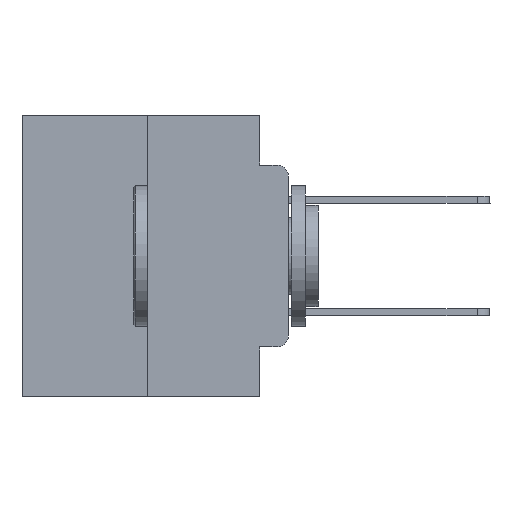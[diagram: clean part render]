
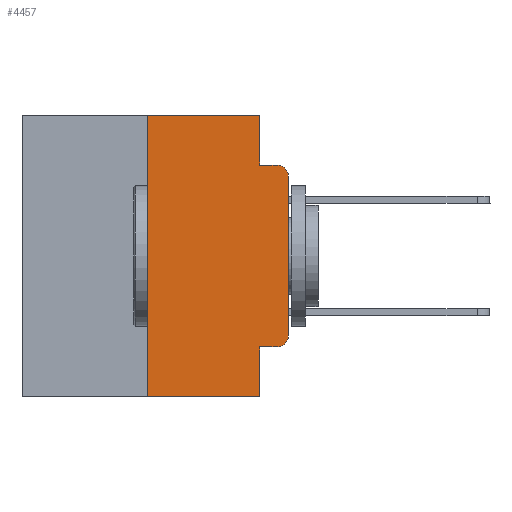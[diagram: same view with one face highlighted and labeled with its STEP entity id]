
A CAD part, left-side view. The second image highlights one B-rep face of the part: STEP entity #4457.
In plain terms, the highlighted planar face has unit normal (-1, 0, 0).
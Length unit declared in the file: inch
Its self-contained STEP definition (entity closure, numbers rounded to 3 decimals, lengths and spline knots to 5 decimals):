
#170 = VECTOR ( 'NONE', #10682, 39.37008 ) ;
#253 = CARTESIAN_POINT ( 'NONE',  ( 0., 0.051, -0.0885 ) ) ;
#426 = CIRCLE ( 'NONE', #10935, 0.02 ) ;
#489 = DIRECTION ( 'NONE',  ( 0., 0., -1. ) ) ;
#490 = ORIENTED_EDGE ( 'NONE', *, *, #3963, .F. ) ;
#1934 = ORIENTED_EDGE ( 'NONE', *, *, #18304, .F. ) ;
#2082 = FACE_OUTER_BOUND ( 'NONE', #13481, .T. ) ;
#2412 = LINE ( 'NONE', #6698, #9205 ) ;
#3065 = DIRECTION ( 'NONE',  ( 0., -1., 0. ) ) ;
#3871 = CARTESIAN_POINT ( 'NONE',  ( 0., 0.051, -0.4115 ) ) ;
#3873 = DIRECTION ( 'NONE',  ( 0., 0., 1. ) ) ;
#3963 = EDGE_CURVE ( 'NONE', #28118, #27911, #18214, .T. ) ;
#4024 = CARTESIAN_POINT ( 'NONE',  ( 0., 0.02, -0.0885 ) ) ;
#4457 = ADVANCED_FACE ( 'NONE', ( #2082 ), #15470, .F. ) ;
#4655 = DIRECTION ( 'NONE',  ( 0., -1., 0. ) ) ;
#4785 = EDGE_CURVE ( 'NONE', #17108, #12115, #7833, .T. ) ;
#4813 = DIRECTION ( 'NONE',  ( 0., 0., -1. ) ) ;
#5510 = ORIENTED_EDGE ( 'NONE', *, *, #4785, .T. ) ;
#5801 = VECTOR ( 'NONE', #9537, 39.37008 ) ;
#5929 = CARTESIAN_POINT ( 'NONE',  ( 0., 0.051, -0.4115 ) ) ;
#5963 = CARTESIAN_POINT ( 'NONE',  ( 0., 0.02, -0.1085 ) ) ;
#6230 = DIRECTION ( 'NONE',  ( 0., 0., -1. ) ) ;
#6346 = LINE ( 'NONE', #23886, #170 ) ;
#6427 = CARTESIAN_POINT ( 'NONE',  ( 0., 0., -0.3915 ) ) ;
#6698 = CARTESIAN_POINT ( 'NONE',  ( 0., 0.051, 0. ) ) ;
#7161 = CARTESIAN_POINT ( 'NONE',  ( 0., 0., 0. ) ) ;
#7327 = EDGE_CURVE ( 'NONE', #15707, #21392, #11937, .T. ) ;
#7483 = VECTOR ( 'NONE', #16942, 39.37008 ) ;
#7833 = LINE ( 'NONE', #7161, #5801 ) ;
#8569 = ORIENTED_EDGE ( 'NONE', *, *, #23806, .F. ) ;
#8581 = VECTOR ( 'NONE', #4655, 39.37008 ) ;
#9099 = CARTESIAN_POINT ( 'NONE',  ( 0., 0.473, 0. ) ) ;
#9205 = VECTOR ( 'NONE', #489, 39.37008 ) ;
#9537 = DIRECTION ( 'NONE',  ( 0., 0., 1. ) ) ;
#9741 = VECTOR ( 'NONE', #12389, 39.37008 ) ;
#9836 = EDGE_CURVE ( 'NONE', #15707, #21250, #27657, .T. ) ;
#9845 = CARTESIAN_POINT ( 'NONE',  ( 0., 0.473, -0.5 ) ) ;
#10579 = EDGE_CURVE ( 'NONE', #12115, #27911, #12468, .T. ) ;
#10682 = DIRECTION ( 'NONE',  ( 0., -1., 0. ) ) ;
#10935 = AXIS2_PLACEMENT_3D ( 'NONE', #25109, #18596, #11920 ) ;
#11128 = VECTOR ( 'NONE', #3873, 39.37008 ) ;
#11257 = EDGE_CURVE ( 'NONE', #21392, #17108, #426, .T. ) ;
#11804 = CARTESIAN_POINT ( 'NONE',  ( 0., 0.25, -0.5 ) ) ;
#11920 = DIRECTION ( 'NONE',  ( 0., 0., -1. ) ) ;
#11937 = LINE ( 'NONE', #3871, #7483 ) ;
#12115 = VERTEX_POINT ( 'NONE', #17594 ) ;
#12389 = DIRECTION ( 'NONE',  ( 0., 0., -1. ) ) ;
#12451 = AXIS2_PLACEMENT_3D ( 'NONE', #5963, #14657, #6230 ) ;
#12468 = CIRCLE ( 'NONE', #12451, 0.02 ) ;
#13207 = EDGE_CURVE ( 'NONE', #23626, #19630, #6346, .T. ) ;
#13481 = EDGE_LOOP ( 'NONE', ( #5510, #17336, #490, #8569, #22310, #1934, #15549, #16975, #15427, #27945 ) ) ;
#14657 = DIRECTION ( 'NONE',  ( -1., 0., 0. ) ) ;
#14857 = EDGE_CURVE ( 'NONE', #16083, #21250, #25503, .T. ) ;
#14900 = CARTESIAN_POINT ( 'NONE',  ( 0., 0.25, 0. ) ) ;
#15427 = ORIENTED_EDGE ( 'NONE', *, *, #7327, .T. ) ;
#15470 = PLANE ( 'NONE',  #24108 ) ;
#15549 = ORIENTED_EDGE ( 'NONE', *, *, #14857, .T. ) ;
#15707 = VERTEX_POINT ( 'NONE', #5929 ) ;
#15742 = DIRECTION ( 'NONE',  ( 1., 0., 0. ) ) ;
#16083 = VERTEX_POINT ( 'NONE', #11804 ) ;
#16942 = DIRECTION ( 'NONE',  ( 0., -1., 0. ) ) ;
#16975 = ORIENTED_EDGE ( 'NONE', *, *, #9836, .F. ) ;
#17108 = VERTEX_POINT ( 'NONE', #6427 ) ;
#17321 = CARTESIAN_POINT ( 'NONE',  ( 0., 0.25, 0. ) ) ;
#17336 = ORIENTED_EDGE ( 'NONE', *, *, #10579, .T. ) ;
#17594 = CARTESIAN_POINT ( 'NONE',  ( 0., 0., -0.1085 ) ) ;
#18214 = LINE ( 'NONE', #253, #8581 ) ;
#18304 = EDGE_CURVE ( 'NONE', #16083, #23626, #18428, .T. ) ;
#18428 = LINE ( 'NONE', #17321, #11128 ) ;
#18596 = DIRECTION ( 'NONE',  ( -1., 0., 0. ) ) ;
#19630 = VERTEX_POINT ( 'NONE', #22324 ) ;
#19947 = CARTESIAN_POINT ( 'NONE',  ( 0., 0.02, -0.4115 ) ) ;
#20229 = CARTESIAN_POINT ( 'NONE',  ( 0., 0.051, -0.0885 ) ) ;
#21250 = VERTEX_POINT ( 'NONE', #27933 ) ;
#21392 = VERTEX_POINT ( 'NONE', #19947 ) ;
#21626 = CARTESIAN_POINT ( 'NONE',  ( 0., 0.051, 0. ) ) ;
#22310 = ORIENTED_EDGE ( 'NONE', *, *, #13207, .F. ) ;
#22324 = CARTESIAN_POINT ( 'NONE',  ( 0., 0.051, 0. ) ) ;
#23067 = VECTOR ( 'NONE', #3065, 39.37008 ) ;
#23626 = VERTEX_POINT ( 'NONE', #14900 ) ;
#23806 = EDGE_CURVE ( 'NONE', #19630, #28118, #2412, .T. ) ;
#23886 = CARTESIAN_POINT ( 'NONE',  ( 0., 0.473, 0. ) ) ;
#24108 = AXIS2_PLACEMENT_3D ( 'NONE', #9099, #15742, #4813 ) ;
#25109 = CARTESIAN_POINT ( 'NONE',  ( 0., 0.02, -0.3915 ) ) ;
#25503 = LINE ( 'NONE', #9845, #23067 ) ;
#27657 = LINE ( 'NONE', #21626, #9741 ) ;
#27911 = VERTEX_POINT ( 'NONE', #4024 ) ;
#27933 = CARTESIAN_POINT ( 'NONE',  ( 0., 0.051, -0.5 ) ) ;
#27945 = ORIENTED_EDGE ( 'NONE', *, *, #11257, .T. ) ;
#28118 = VERTEX_POINT ( 'NONE', #20229 ) ;
